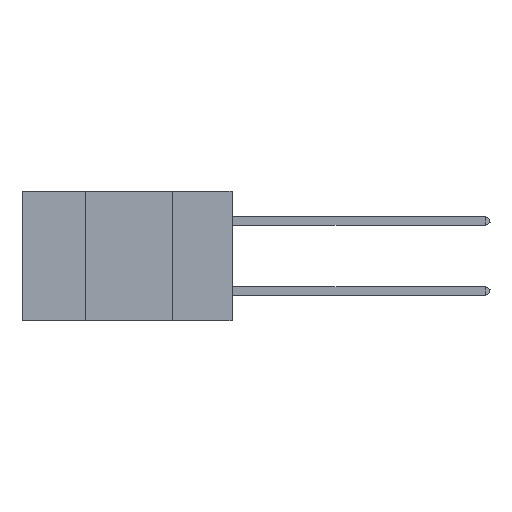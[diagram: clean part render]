
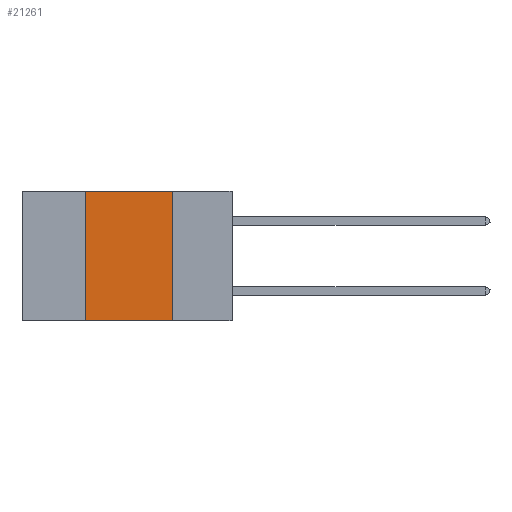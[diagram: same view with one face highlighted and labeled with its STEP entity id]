
A CAD part, left-side view. The second image highlights one B-rep face of the part: STEP entity #21261.
In plain terms, the highlighted planar face has unit normal (-1, 0, 0).
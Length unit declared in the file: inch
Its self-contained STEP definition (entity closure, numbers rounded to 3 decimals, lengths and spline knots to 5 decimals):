
#77 = CARTESIAN_POINT ( 'NONE',  ( 0., 0.17, -0.37 ) ) ;
#525 = DIRECTION ( 'NONE',  ( 0., -1., 0. ) ) ;
#530 = VERTEX_POINT ( 'NONE', #20672 ) ;
#3006 = CARTESIAN_POINT ( 'NONE',  ( 0., 0.6, -0.37 ) ) ;
#5342 = CARTESIAN_POINT ( 'NONE',  ( 0., 0.6, 0. ) ) ;
#7188 = VECTOR ( 'NONE', #35100, 39.37008 ) ;
#8353 = DIRECTION ( 'NONE',  ( 1., 0., 0. ) ) ;
#8494 = DIRECTION ( 'NONE',  ( 0., -1., 0. ) ) ;
#11325 = CARTESIAN_POINT ( 'NONE',  ( 0., 0.42, -0.37 ) ) ;
#11340 = EDGE_LOOP ( 'NONE', ( #18156, #11453, #16394, #19933 ) ) ;
#11453 = ORIENTED_EDGE ( 'NONE', *, *, #25694, .F. ) ;
#11799 = EDGE_CURVE ( 'NONE', #11864, #20531, #20648, .T. ) ;
#11864 = VERTEX_POINT ( 'NONE', #11325 ) ;
#13750 = DIRECTION ( 'NONE',  ( 0., 0., -1. ) ) ;
#16394 = ORIENTED_EDGE ( 'NONE', *, *, #35767, .F. ) ;
#16662 = VECTOR ( 'NONE', #8494, 39.37008 ) ;
#18156 = ORIENTED_EDGE ( 'NONE', *, *, #34856, .F. ) ;
#19933 = ORIENTED_EDGE ( 'NONE', *, *, #11799, .T. ) ;
#20531 = VERTEX_POINT ( 'NONE', #77 ) ;
#20648 = LINE ( 'NONE', #3006, #16662 ) ;
#20672 = CARTESIAN_POINT ( 'NONE',  ( 0., 0.17, 0. ) ) ;
#21261 = ADVANCED_FACE ( 'NONE', ( #21456 ), #25357, .F. ) ;
#21456 = FACE_OUTER_BOUND ( 'NONE', #11340, .T. ) ;
#25357 = PLANE ( 'NONE',  #29114 ) ;
#25694 = EDGE_CURVE ( 'NONE', #35753, #530, #34133, .T. ) ;
#29114 = AXIS2_PLACEMENT_3D ( 'NONE', #5342, #8353, #31076 ) ;
#29725 = CARTESIAN_POINT ( 'NONE',  ( 0., 0.42, 0. ) ) ;
#30779 = CARTESIAN_POINT ( 'NONE',  ( 0., 0.17, 0. ) ) ;
#31076 = DIRECTION ( 'NONE',  ( 0., 0., -1. ) ) ;
#32771 = VECTOR ( 'NONE', #525, 39.37008 ) ;
#33452 = LINE ( 'NONE', #29725, #7188 ) ;
#33518 = LINE ( 'NONE', #30779, #35316 ) ;
#34133 = LINE ( 'NONE', #34830, #32771 ) ;
#34830 = CARTESIAN_POINT ( 'NONE',  ( 0., 0.6, 0. ) ) ;
#34856 = EDGE_CURVE ( 'NONE', #530, #20531, #33518, .T. ) ;
#35100 = DIRECTION ( 'NONE',  ( 0., 0., 1. ) ) ;
#35222 = CARTESIAN_POINT ( 'NONE',  ( 0., 0.42, 0. ) ) ;
#35316 = VECTOR ( 'NONE', #13750, 39.37008 ) ;
#35753 = VERTEX_POINT ( 'NONE', #35222 ) ;
#35767 = EDGE_CURVE ( 'NONE', #11864, #35753, #33452, .T. ) ;
